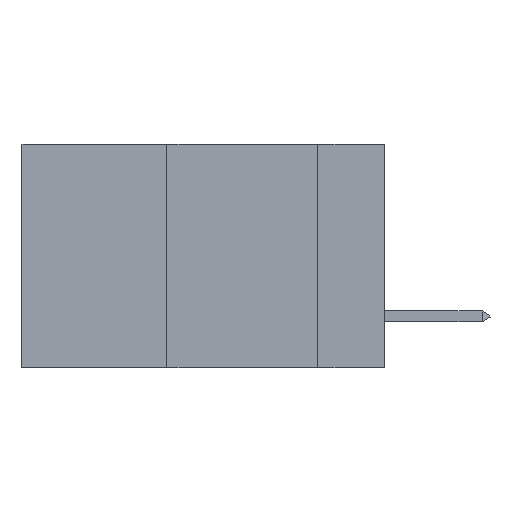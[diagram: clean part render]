
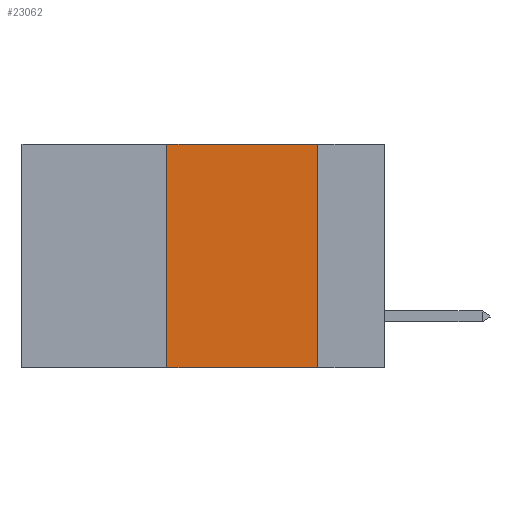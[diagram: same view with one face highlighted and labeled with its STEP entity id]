
A CAD part, left-side view. The second image highlights one B-rep face of the part: STEP entity #23062.
In plain terms, the highlighted planar face has unit normal (-1, 0, 0).
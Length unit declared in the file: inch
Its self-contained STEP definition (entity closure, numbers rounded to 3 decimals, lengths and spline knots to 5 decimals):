
#102 = EDGE_LOOP ( 'NONE', ( #8622, #20824, #36465, #2637 ) ) ;
#259 = VECTOR ( 'NONE', #9646, 39.37008 ) ;
#2637 = ORIENTED_EDGE ( 'NONE', *, *, #50661, .T. ) ;
#3414 = CARTESIAN_POINT ( 'NONE',  ( 0., 0.36, 0. ) ) ;
#5040 = CARTESIAN_POINT ( 'NONE',  ( 0., 0.11, 0. ) ) ;
#6260 = CARTESIAN_POINT ( 'NONE',  ( 0., 0.6, -0.37 ) ) ;
#8132 = VERTEX_POINT ( 'NONE', #18068 ) ;
#8622 = ORIENTED_EDGE ( 'NONE', *, *, #15990, .F. ) ;
#9646 = DIRECTION ( 'NONE',  ( 0., -1., 0. ) ) ;
#10350 = VECTOR ( 'NONE', #38146, 39.37008 ) ;
#10783 = LINE ( 'NONE', #6260, #259 ) ;
#13368 = LINE ( 'NONE', #3414, #10350 ) ;
#13393 = DIRECTION ( 'NONE',  ( 1., 0., 0. ) ) ;
#15990 = EDGE_CURVE ( 'NONE', #35341, #8132, #47222, .T. ) ;
#18068 = CARTESIAN_POINT ( 'NONE',  ( 0., 0.11, -0.37 ) ) ;
#19630 = VERTEX_POINT ( 'NONE', #48403 ) ;
#20824 = ORIENTED_EDGE ( 'NONE', *, *, #30147, .F. ) ;
#20939 = CARTESIAN_POINT ( 'NONE',  ( 0., 0.6, 0. ) ) ;
#23062 = ADVANCED_FACE ( 'NONE', ( #42484 ), #37024, .F. ) ;
#25157 = VERTEX_POINT ( 'NONE', #29799 ) ;
#26307 = VECTOR ( 'NONE', #49879, 39.37008 ) ;
#28584 = CARTESIAN_POINT ( 'NONE',  ( 0., 0.6, 0. ) ) ;
#29481 = DIRECTION ( 'NONE',  ( 0., -1., 0. ) ) ;
#29799 = CARTESIAN_POINT ( 'NONE',  ( 0., 0.36, -0.37 ) ) ;
#30147 = EDGE_CURVE ( 'NONE', #19630, #35341, #49962, .T. ) ;
#35341 = VERTEX_POINT ( 'NONE', #5040 ) ;
#36465 = ORIENTED_EDGE ( 'NONE', *, *, #43195, .F. ) ;
#37024 = PLANE ( 'NONE',  #46475 ) ;
#38146 = DIRECTION ( 'NONE',  ( 0., 0., 1. ) ) ;
#39500 = VECTOR ( 'NONE', #29481, 39.37008 ) ;
#41432 = CARTESIAN_POINT ( 'NONE',  ( 0., 0.11, 0. ) ) ;
#42484 = FACE_OUTER_BOUND ( 'NONE', #102, .T. ) ;
#43195 = EDGE_CURVE ( 'NONE', #25157, #19630, #13368, .T. ) ;
#46475 = AXIS2_PLACEMENT_3D ( 'NONE', #20939, #13393, #48996 ) ;
#47222 = LINE ( 'NONE', #41432, #26307 ) ;
#48403 = CARTESIAN_POINT ( 'NONE',  ( 0., 0.36, 0. ) ) ;
#48996 = DIRECTION ( 'NONE',  ( 0., 0., -1. ) ) ;
#49879 = DIRECTION ( 'NONE',  ( 0., 0., -1. ) ) ;
#49962 = LINE ( 'NONE', #28584, #39500 ) ;
#50661 = EDGE_CURVE ( 'NONE', #25157, #8132, #10783, .T. ) ;
